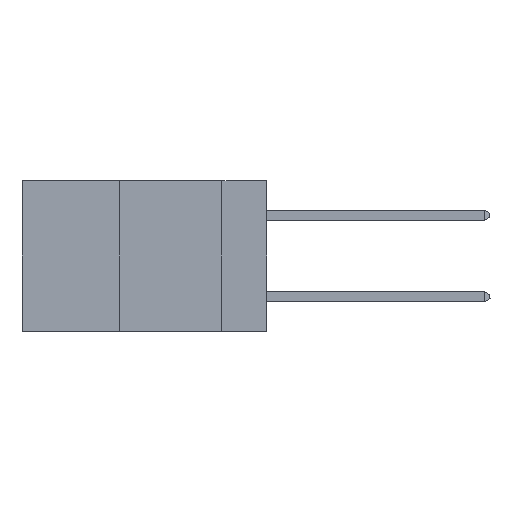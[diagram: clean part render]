
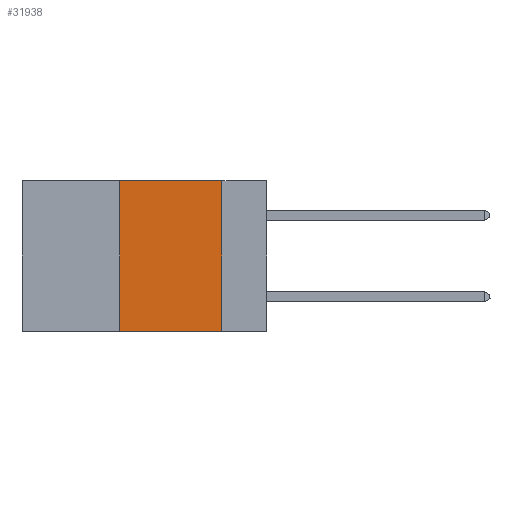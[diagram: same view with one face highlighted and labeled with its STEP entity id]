
A CAD part, left-side view. The second image highlights one B-rep face of the part: STEP entity #31938.
In plain terms, the highlighted planar face has unit normal (-1, 0, 0).
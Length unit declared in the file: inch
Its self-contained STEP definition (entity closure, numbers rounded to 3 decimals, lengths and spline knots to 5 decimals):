
#698 = VECTOR ( 'NONE', #3134, 39.37008 ) ;
#1284 = CARTESIAN_POINT ( 'NONE',  ( 0., 0.6, 0. ) ) ;
#2443 = CARTESIAN_POINT ( 'NONE',  ( 0., 0.36, -0.37 ) ) ;
#3134 = DIRECTION ( 'NONE',  ( 0., -1., 0. ) ) ;
#7375 = CARTESIAN_POINT ( 'NONE',  ( 0., 0.36, 0. ) ) ;
#7442 = VECTOR ( 'NONE', #10525, 39.37008 ) ;
#8988 = CARTESIAN_POINT ( 'NONE',  ( 0., 0.6, 0. ) ) ;
#9120 = PLANE ( 'NONE',  #19396 ) ;
#9873 = EDGE_CURVE ( 'NONE', #26433, #30405, #39456, .T. ) ;
#10525 = DIRECTION ( 'NONE',  ( 0., 0., -1. ) ) ;
#10602 = ORIENTED_EDGE ( 'NONE', *, *, #32337, .F. ) ;
#11813 = VECTOR ( 'NONE', #31677, 39.37008 ) ;
#15271 = VECTOR ( 'NONE', #31831, 39.37008 ) ;
#15514 = ORIENTED_EDGE ( 'NONE', *, *, #38823, .F. ) ;
#17030 = CARTESIAN_POINT ( 'NONE',  ( 0., 0.11, -0.37 ) ) ;
#18136 = LINE ( 'NONE', #7375, #15271 ) ;
#18174 = CARTESIAN_POINT ( 'NONE',  ( 0., 0.36, 0. ) ) ;
#18643 = FACE_OUTER_BOUND ( 'NONE', #33094, .T. ) ;
#19396 = AXIS2_PLACEMENT_3D ( 'NONE', #8988, #33701, #27532 ) ;
#25437 = ORIENTED_EDGE ( 'NONE', *, *, #9873, .F. ) ;
#26433 = VERTEX_POINT ( 'NONE', #35124 ) ;
#27532 = DIRECTION ( 'NONE',  ( 0., 0., -1. ) ) ;
#29163 = CARTESIAN_POINT ( 'NONE',  ( 0., 0.11, 0. ) ) ;
#29419 = LINE ( 'NONE', #1284, #11813 ) ;
#30405 = VERTEX_POINT ( 'NONE', #17030 ) ;
#31677 = DIRECTION ( 'NONE',  ( 0., -1., 0. ) ) ;
#31831 = DIRECTION ( 'NONE',  ( 0., 0., 1. ) ) ;
#31938 = ADVANCED_FACE ( 'NONE', ( #18643 ), #9120, .F. ) ;
#32337 = EDGE_CURVE ( 'NONE', #33192, #33818, #18136, .T. ) ;
#33094 = EDGE_LOOP ( 'NONE', ( #25437, #15514, #10602, #39457 ) ) ;
#33192 = VERTEX_POINT ( 'NONE', #2443 ) ;
#33701 = DIRECTION ( 'NONE',  ( 1., 0., 0. ) ) ;
#33793 = CARTESIAN_POINT ( 'NONE',  ( 0., 0.6, -0.37 ) ) ;
#33818 = VERTEX_POINT ( 'NONE', #18174 ) ;
#35124 = CARTESIAN_POINT ( 'NONE',  ( 0., 0.11, 0. ) ) ;
#36122 = LINE ( 'NONE', #33793, #698 ) ;
#38823 = EDGE_CURVE ( 'NONE', #33818, #26433, #29419, .T. ) ;
#39258 = EDGE_CURVE ( 'NONE', #33192, #30405, #36122, .T. ) ;
#39456 = LINE ( 'NONE', #29163, #7442 ) ;
#39457 = ORIENTED_EDGE ( 'NONE', *, *, #39258, .T. ) ;
